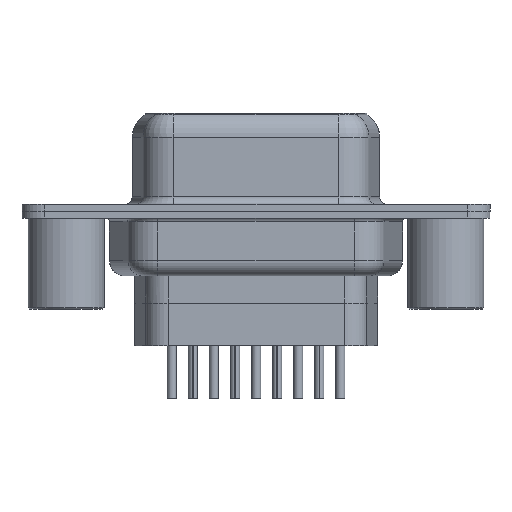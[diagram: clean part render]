
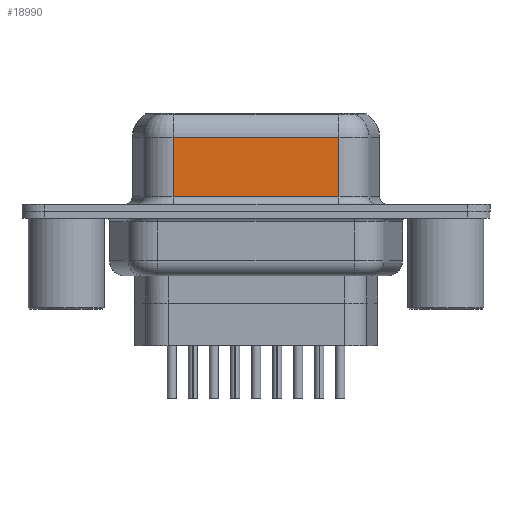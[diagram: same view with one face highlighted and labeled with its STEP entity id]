
A CAD part, front view. The second image highlights one B-rep face of the part: STEP entity #18990.
In plain terms, the highlighted planar face has unit normal (0, -1, 0).
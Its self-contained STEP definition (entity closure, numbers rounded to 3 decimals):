
#1008 = VECTOR ( 'NONE', #13306, 1000. ) ;
#1510 = ORIENTED_EDGE ( 'NONE', *, *, #18331, .F. ) ;
#3039 = EDGE_CURVE ( 'NONE', #10880, #6819, #16488, .T. ) ;
#3170 = AXIS2_PLACEMENT_3D ( 'NONE', #4410, #6274, #22423 ) ;
#3746 = ORIENTED_EDGE ( 'NONE', *, *, #20804, .T. ) ;
#4291 = VECTOR ( 'NONE', #7441, 1000. ) ;
#4410 = CARTESIAN_POINT ( 'NONE',  ( 17.957, -3.95, 6.6 ) ) ;
#4676 = CARTESIAN_POINT ( 'NONE',  ( 17.957, -3.95, 4.85 ) ) ;
#6192 = VERTEX_POINT ( 'NONE', #4676 ) ;
#6274 = DIRECTION ( 'NONE',  ( 0., 1., 0. ) ) ;
#6819 = VERTEX_POINT ( 'NONE', #14973 ) ;
#7441 = DIRECTION ( 'NONE',  ( -1., 0., 0. ) ) ;
#8911 = DIRECTION ( 'NONE',  ( 0., 0., -1. ) ) ;
#9302 = ORIENTED_EDGE ( 'NONE', *, *, #3039, .T. ) ;
#10880 = VERTEX_POINT ( 'NONE', #22822 ) ;
#10974 = LINE ( 'NONE', #16738, #4291 ) ;
#13247 = FACE_OUTER_BOUND ( 'NONE', #13461, .T. ) ;
#13306 = DIRECTION ( 'NONE',  ( 1., 0., 0. ) ) ;
#13461 = EDGE_LOOP ( 'NONE', ( #1510, #22361, #3746, #9302 ) ) ;
#14498 = VECTOR ( 'NONE', #19918, 1000. ) ;
#14825 = CARTESIAN_POINT ( 'NONE',  ( 7.033, -3.95, 6.6 ) ) ;
#14973 = CARTESIAN_POINT ( 'NONE',  ( 17.957, -3.95, 0.95 ) ) ;
#15740 = VERTEX_POINT ( 'NONE', #22224 ) ;
#16488 = LINE ( 'NONE', #22259, #1008 ) ;
#16738 = CARTESIAN_POINT ( 'NONE',  ( 17.957, -3.95, 4.85 ) ) ;
#17498 = EDGE_CURVE ( 'NONE', #6192, #15740, #10974, .T. ) ;
#18331 = EDGE_CURVE ( 'NONE', #6192, #6819, #21888, .T. ) ;
#18466 = CARTESIAN_POINT ( 'NONE',  ( 17.957, -3.95, 6.6 ) ) ;
#18990 = ADVANCED_FACE ( 'NONE', ( #13247 ), #20544, .F. ) ;
#19374 = VECTOR ( 'NONE', #8911, 1000. ) ;
#19918 = DIRECTION ( 'NONE',  ( 0., 0., -1. ) ) ;
#20259 = LINE ( 'NONE', #14825, #14498 ) ;
#20544 = PLANE ( 'NONE',  #3170 ) ;
#20804 = EDGE_CURVE ( 'NONE', #15740, #10880, #20259, .T. ) ;
#21888 = LINE ( 'NONE', #18466, #19374 ) ;
#22224 = CARTESIAN_POINT ( 'NONE',  ( 7.033, -3.95, 4.85 ) ) ;
#22259 = CARTESIAN_POINT ( 'NONE',  ( 17.957, -3.95, 0.95 ) ) ;
#22361 = ORIENTED_EDGE ( 'NONE', *, *, #17498, .T. ) ;
#22423 = DIRECTION ( 'NONE',  ( 0., 0., 1. ) ) ;
#22822 = CARTESIAN_POINT ( 'NONE',  ( 7.033, -3.95, 0.95 ) ) ;
